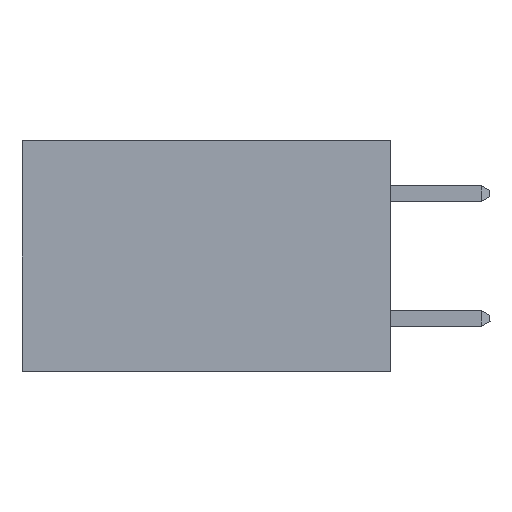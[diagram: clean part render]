
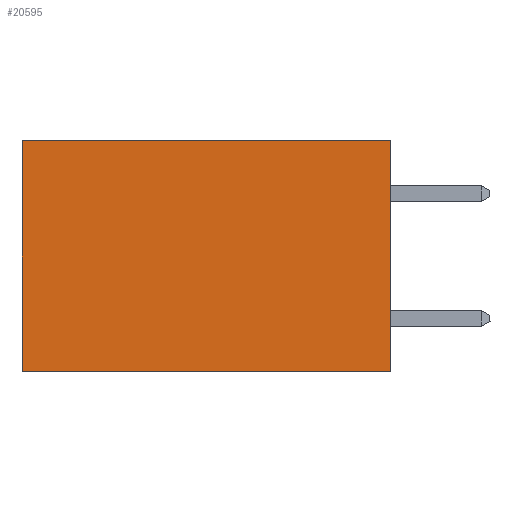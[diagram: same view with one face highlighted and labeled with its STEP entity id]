
A CAD part, left-side view. The second image highlights one B-rep face of the part: STEP entity #20595.
In plain terms, the highlighted planar face has unit normal (-1, 0, 0).
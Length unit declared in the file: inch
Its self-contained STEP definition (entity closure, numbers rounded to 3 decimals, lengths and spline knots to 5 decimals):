
#753 = LINE ( 'NONE', #10826, #19524 ) ;
#1232 = VECTOR ( 'NONE', #17224, 39.37008 ) ;
#2819 = EDGE_CURVE ( 'NONE', #15270, #4792, #15751, .T. ) ;
#3613 = ORIENTED_EDGE ( 'NONE', *, *, #15098, .T. ) ;
#4094 = LINE ( 'NONE', #23097, #18048 ) ;
#4792 = VERTEX_POINT ( 'NONE', #10986 ) ;
#5098 = PLANE ( 'NONE',  #19032 ) ;
#5119 = FACE_OUTER_BOUND ( 'NONE', #13451, .T. ) ;
#6208 = CARTESIAN_POINT ( 'NONE',  ( 0.277, 0., 0. ) ) ;
#6337 = ORIENTED_EDGE ( 'NONE', *, *, #2819, .T. ) ;
#7628 = ORIENTED_EDGE ( 'NONE', *, *, #12625, .F. ) ;
#8813 = VECTOR ( 'NONE', #16787, 39.37008 ) ;
#8817 = CARTESIAN_POINT ( 'NONE',  ( 0.277, 0., -0.37 ) ) ;
#9016 = CARTESIAN_POINT ( 'NONE',  ( 0.277, 0.59, 0. ) ) ;
#9866 = EDGE_CURVE ( 'NONE', #22628, #17260, #753, .T. ) ;
#10664 = ORIENTED_EDGE ( 'NONE', *, *, #9866, .F. ) ;
#10700 = DIRECTION ( 'NONE',  ( 0., 0., -1. ) ) ;
#10812 = CARTESIAN_POINT ( 'NONE',  ( 0.277, 0., -0.37 ) ) ;
#10826 = CARTESIAN_POINT ( 'NONE',  ( 0.277, 0., -0.37 ) ) ;
#10986 = CARTESIAN_POINT ( 'NONE',  ( 0.277, 0.59, -0.37 ) ) ;
#12625 = EDGE_CURVE ( 'NONE', #17260, #4792, #23335, .T. ) ;
#13451 = EDGE_LOOP ( 'NONE', ( #6337, #7628, #10664, #3613 ) ) ;
#15098 = EDGE_CURVE ( 'NONE', #22628, #15270, #4094, .T. ) ;
#15270 = VERTEX_POINT ( 'NONE', #9016 ) ;
#15751 = LINE ( 'NONE', #23192, #1232 ) ;
#15839 = DIRECTION ( 'NONE',  ( 0., 1., 0. ) ) ;
#16787 = DIRECTION ( 'NONE',  ( 0., 1., 0. ) ) ;
#17224 = DIRECTION ( 'NONE',  ( 0., 0., -1. ) ) ;
#17260 = VERTEX_POINT ( 'NONE', #10812 ) ;
#18048 = VECTOR ( 'NONE', #15839, 39.37008 ) ;
#18058 = DIRECTION ( 'NONE',  ( 0., 0., -1. ) ) ;
#19032 = AXIS2_PLACEMENT_3D ( 'NONE', #8817, #21534, #10700 ) ;
#19524 = VECTOR ( 'NONE', #18058, 39.37008 ) ;
#20595 = ADVANCED_FACE ( 'NONE', ( #5119 ), #5098, .F. ) ;
#21534 = DIRECTION ( 'NONE',  ( 1., 0., 0. ) ) ;
#22309 = CARTESIAN_POINT ( 'NONE',  ( 0.277, 0., -0.37 ) ) ;
#22628 = VERTEX_POINT ( 'NONE', #6208 ) ;
#23097 = CARTESIAN_POINT ( 'NONE',  ( 0.277, 0., 0. ) ) ;
#23192 = CARTESIAN_POINT ( 'NONE',  ( 0.277, 0.59, -0.37 ) ) ;
#23335 = LINE ( 'NONE', #22309, #8813 ) ;
